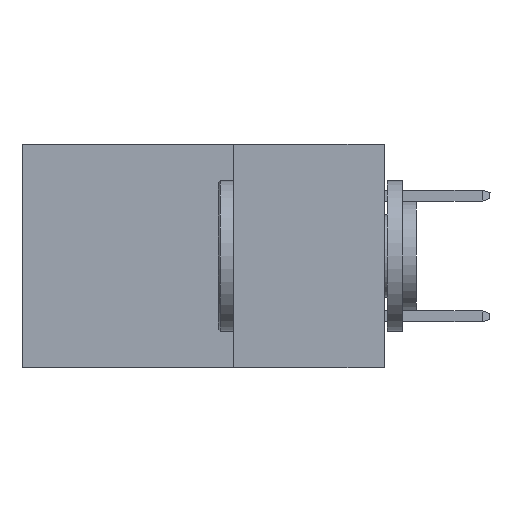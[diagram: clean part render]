
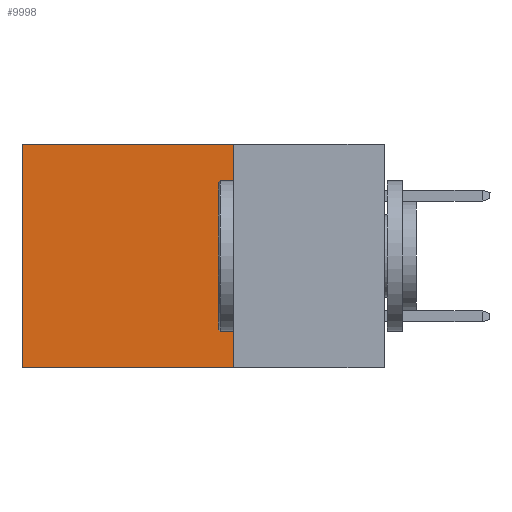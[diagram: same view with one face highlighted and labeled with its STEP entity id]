
A CAD part, left-side view. The second image highlights one B-rep face of the part: STEP entity #9998.
In plain terms, the highlighted planar face has unit normal (-1, 0, 0).
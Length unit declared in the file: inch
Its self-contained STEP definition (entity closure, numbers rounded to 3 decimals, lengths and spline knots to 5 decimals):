
#417 = VERTEX_POINT ( 'NONE', #10575 ) ;
#505 = AXIS2_PLACEMENT_3D ( 'NONE', #8615, #719, #1865 ) ;
#719 = DIRECTION ( 'NONE',  ( 1., 0., 0. ) ) ;
#802 = VECTOR ( 'NONE', #6580, 39.37008 ) ;
#924 = VECTOR ( 'NONE', #14339, 39.37008 ) ;
#1865 = DIRECTION ( 'NONE',  ( 0., 0., -1. ) ) ;
#2067 = EDGE_CURVE ( 'NONE', #3478, #417, #10518, .T. ) ;
#2307 = DIRECTION ( 'NONE',  ( 0., 0., -1. ) ) ;
#2646 = ORIENTED_EDGE ( 'NONE', *, *, #2067, .T. ) ;
#3104 = PLANE ( 'NONE',  #505 ) ;
#3203 = CARTESIAN_POINT ( 'NONE',  ( 0.298, 0.25, -0.37 ) ) ;
#3478 = VERTEX_POINT ( 'NONE', #5735 ) ;
#4569 = VERTEX_POINT ( 'NONE', #10277 ) ;
#4873 = ORIENTED_EDGE ( 'NONE', *, *, #8880, .F. ) ;
#5735 = CARTESIAN_POINT ( 'NONE',  ( 0.298, 0.25, 0. ) ) ;
#5914 = LINE ( 'NONE', #3203, #924 ) ;
#5965 = LINE ( 'NONE', #12633, #13450 ) ;
#6104 = CARTESIAN_POINT ( 'NONE',  ( 0.298, 0.25, 0. ) ) ;
#6387 = EDGE_LOOP ( 'NONE', ( #13513, #4873, #9628, #2646 ) ) ;
#6580 = DIRECTION ( 'NONE',  ( 0., 1., 0. ) ) ;
#6659 = EDGE_CURVE ( 'NONE', #417, #4569, #10714, .T. ) ;
#7440 = EDGE_CURVE ( 'NONE', #3478, #8340, #5965, .T. ) ;
#8340 = VERTEX_POINT ( 'NONE', #13454 ) ;
#8615 = CARTESIAN_POINT ( 'NONE',  ( 0.298, 0.25, 0. ) ) ;
#8880 = EDGE_CURVE ( 'NONE', #8340, #4569, #5914, .T. ) ;
#9628 = ORIENTED_EDGE ( 'NONE', *, *, #7440, .F. ) ;
#9998 = ADVANCED_FACE ( 'NONE', ( #12183 ), #3104, .F. ) ;
#10277 = CARTESIAN_POINT ( 'NONE',  ( 0.298, 0.6, -0.37 ) ) ;
#10364 = VECTOR ( 'NONE', #2307, 39.37008 ) ;
#10518 = LINE ( 'NONE', #6104, #802 ) ;
#10575 = CARTESIAN_POINT ( 'NONE',  ( 0.298, 0.6, 0. ) ) ;
#10714 = LINE ( 'NONE', #12373, #10364 ) ;
#12183 = FACE_OUTER_BOUND ( 'NONE', #6387, .T. ) ;
#12373 = CARTESIAN_POINT ( 'NONE',  ( 0.298, 0.6, 0. ) ) ;
#12633 = CARTESIAN_POINT ( 'NONE',  ( 0.298, 0.25, 0. ) ) ;
#13450 = VECTOR ( 'NONE', #13955, 39.37008 ) ;
#13454 = CARTESIAN_POINT ( 'NONE',  ( 0.298, 0.25, -0.37 ) ) ;
#13513 = ORIENTED_EDGE ( 'NONE', *, *, #6659, .T. ) ;
#13955 = DIRECTION ( 'NONE',  ( 0., 0., -1. ) ) ;
#14339 = DIRECTION ( 'NONE',  ( 0., 1., 0. ) ) ;
